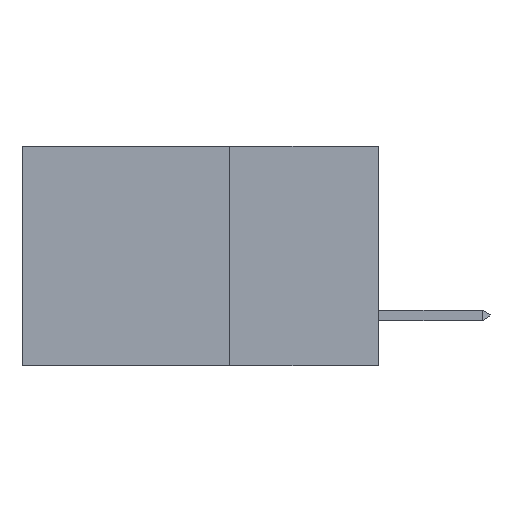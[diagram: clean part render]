
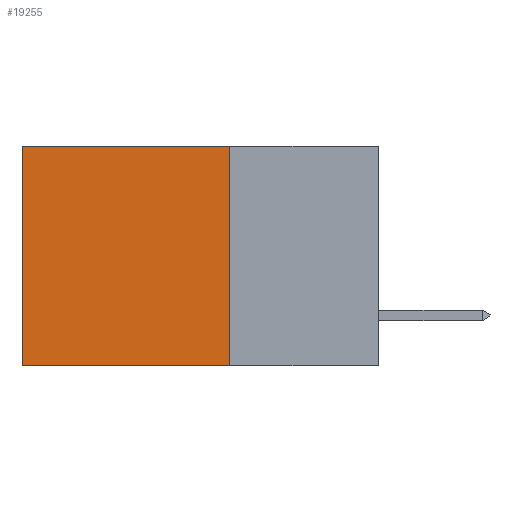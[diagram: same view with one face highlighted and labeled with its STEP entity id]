
A CAD part, left-side view. The second image highlights one B-rep face of the part: STEP entity #19255.
In plain terms, the highlighted planar face has unit normal (-1, 0, 0).
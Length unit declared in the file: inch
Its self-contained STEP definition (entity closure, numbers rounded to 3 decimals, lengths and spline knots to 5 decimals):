
#368 = CARTESIAN_POINT ( 'NONE',  ( 0.298, 0.25, 0. ) ) ;
#1623 = DIRECTION ( 'NONE',  ( 0., 1., 0. ) ) ;
#3791 = VERTEX_POINT ( 'NONE', #23300 ) ;
#4838 = ORIENTED_EDGE ( 'NONE', *, *, #6527, .F. ) ;
#5229 = DIRECTION ( 'NONE',  ( 0., 0., -1. ) ) ;
#5235 = LINE ( 'NONE', #12444, #27736 ) ;
#5837 = VERTEX_POINT ( 'NONE', #18341 ) ;
#5967 = LINE ( 'NONE', #6112, #14812 ) ;
#6112 = CARTESIAN_POINT ( 'NONE',  ( 0.298, 0.25, -0.37 ) ) ;
#6146 = ORIENTED_EDGE ( 'NONE', *, *, #23928, .T. ) ;
#6527 = EDGE_CURVE ( 'NONE', #3791, #26865, #5967, .T. ) ;
#6854 = PLANE ( 'NONE',  #22008 ) ;
#7006 = ORIENTED_EDGE ( 'NONE', *, *, #27333, .T. ) ;
#8486 = LINE ( 'NONE', #18264, #16298 ) ;
#9301 = CARTESIAN_POINT ( 'NONE',  ( 0.298, 0.25, 0. ) ) ;
#11342 = EDGE_CURVE ( 'NONE', #19150, #3791, #8486, .T. ) ;
#12444 = CARTESIAN_POINT ( 'NONE',  ( 0.298, 0.25, 0. ) ) ;
#13220 = CARTESIAN_POINT ( 'NONE',  ( 0.298, 0.6, 0. ) ) ;
#14812 = VECTOR ( 'NONE', #17732, 39.37008 ) ;
#15909 = LINE ( 'NONE', #13220, #18325 ) ;
#16298 = VECTOR ( 'NONE', #5229, 39.37008 ) ;
#17492 = EDGE_LOOP ( 'NONE', ( #6146, #4838, #23655, #7006 ) ) ;
#17732 = DIRECTION ( 'NONE',  ( 0., 1., 0. ) ) ;
#17792 = DIRECTION ( 'NONE',  ( 1., 0., 0. ) ) ;
#18264 = CARTESIAN_POINT ( 'NONE',  ( 0.298, 0.25, 0. ) ) ;
#18325 = VECTOR ( 'NONE', #19706, 39.37008 ) ;
#18341 = CARTESIAN_POINT ( 'NONE',  ( 0.298, 0.6, 0. ) ) ;
#18581 = FACE_OUTER_BOUND ( 'NONE', #17492, .T. ) ;
#19150 = VERTEX_POINT ( 'NONE', #9301 ) ;
#19255 = ADVANCED_FACE ( 'NONE', ( #18581 ), #6854, .F. ) ;
#19706 = DIRECTION ( 'NONE',  ( 0., 0., -1. ) ) ;
#20254 = DIRECTION ( 'NONE',  ( 0., 0., -1. ) ) ;
#21901 = CARTESIAN_POINT ( 'NONE',  ( 0.298, 0.6, -0.37 ) ) ;
#22008 = AXIS2_PLACEMENT_3D ( 'NONE', #368, #17792, #20254 ) ;
#23300 = CARTESIAN_POINT ( 'NONE',  ( 0.298, 0.25, -0.37 ) ) ;
#23655 = ORIENTED_EDGE ( 'NONE', *, *, #11342, .F. ) ;
#23928 = EDGE_CURVE ( 'NONE', #5837, #26865, #15909, .T. ) ;
#26865 = VERTEX_POINT ( 'NONE', #21901 ) ;
#27333 = EDGE_CURVE ( 'NONE', #19150, #5837, #5235, .T. ) ;
#27736 = VECTOR ( 'NONE', #1623, 39.37008 ) ;
